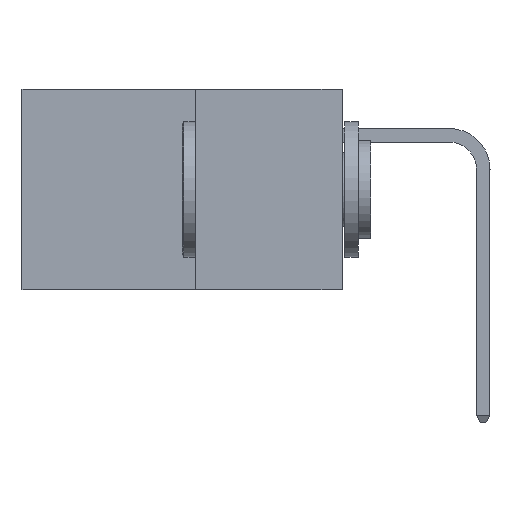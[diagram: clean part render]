
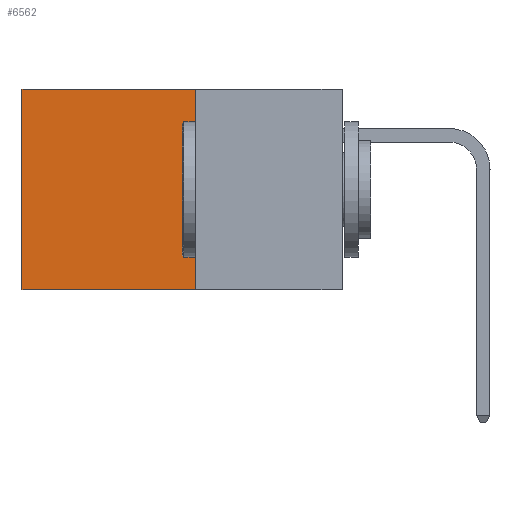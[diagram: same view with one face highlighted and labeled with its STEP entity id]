
A CAD part, left-side view. The second image highlights one B-rep face of the part: STEP entity #6562.
In plain terms, the highlighted planar face has unit normal (-1, 0, 0).
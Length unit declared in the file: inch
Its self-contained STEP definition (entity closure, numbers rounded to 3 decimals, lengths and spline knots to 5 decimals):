
#25 = CARTESIAN_POINT ( 'NONE',  ( 0.277, 0.27, -0.37 ) ) ;
#29 = LINE ( 'NONE', #4669, #7481 ) ;
#82 = DIRECTION ( 'NONE',  ( 0., 0., -1. ) ) ;
#165 = LINE ( 'NONE', #6528, #9218 ) ;
#208 = CARTESIAN_POINT ( 'NONE',  ( 0.277, 0.27, 0. ) ) ;
#1221 = VERTEX_POINT ( 'NONE', #7342 ) ;
#1518 = ORIENTED_EDGE ( 'NONE', *, *, #8991, .F. ) ;
#1585 = CARTESIAN_POINT ( 'NONE',  ( 0.277, 0.27, -0.37 ) ) ;
#2107 = CARTESIAN_POINT ( 'NONE',  ( 0.277, 0.59, -0.37 ) ) ;
#2248 = CARTESIAN_POINT ( 'NONE',  ( 0.277, 0.59, 0. ) ) ;
#2846 = CARTESIAN_POINT ( 'NONE',  ( 0.277, 0.59, -0.37 ) ) ;
#2907 = EDGE_CURVE ( 'NONE', #7593, #7611, #29, .T. ) ;
#4214 = EDGE_CURVE ( 'NONE', #1221, #11573, #5354, .T. ) ;
#4432 = DIRECTION ( 'NONE',  ( 1., 0., 0. ) ) ;
#4669 = CARTESIAN_POINT ( 'NONE',  ( 0.277, 0.27, 0. ) ) ;
#5060 = DIRECTION ( 'NONE',  ( 0., 1., 0. ) ) ;
#5354 = LINE ( 'NONE', #25, #7894 ) ;
#5615 = DIRECTION ( 'NONE',  ( 0., 0., -1. ) ) ;
#5915 = VECTOR ( 'NONE', #82, 39.37008 ) ;
#6528 = CARTESIAN_POINT ( 'NONE',  ( 0.277, 0.27, -0.37 ) ) ;
#6562 = ADVANCED_FACE ( 'NONE', ( #10957 ), #10112, .F. ) ;
#7342 = CARTESIAN_POINT ( 'NONE',  ( 0.277, 0.27, -0.37 ) ) ;
#7481 = VECTOR ( 'NONE', #5060, 39.37008 ) ;
#7593 = VERTEX_POINT ( 'NONE', #208 ) ;
#7611 = VERTEX_POINT ( 'NONE', #2248 ) ;
#7814 = ORIENTED_EDGE ( 'NONE', *, *, #2907, .T. ) ;
#7894 = VECTOR ( 'NONE', #9561, 39.37008 ) ;
#8294 = ORIENTED_EDGE ( 'NONE', *, *, #9733, .T. ) ;
#8991 = EDGE_CURVE ( 'NONE', #7593, #1221, #165, .T. ) ;
#9030 = EDGE_LOOP ( 'NONE', ( #8294, #11590, #1518, #7814 ) ) ;
#9218 = VECTOR ( 'NONE', #5615, 39.37008 ) ;
#9561 = DIRECTION ( 'NONE',  ( 0., 1., 0. ) ) ;
#9733 = EDGE_CURVE ( 'NONE', #7611, #11573, #10869, .T. ) ;
#10112 = PLANE ( 'NONE',  #12219 ) ;
#10869 = LINE ( 'NONE', #2107, #5915 ) ;
#10957 = FACE_OUTER_BOUND ( 'NONE', #9030, .T. ) ;
#11003 = DIRECTION ( 'NONE',  ( 0., 0., -1. ) ) ;
#11573 = VERTEX_POINT ( 'NONE', #2846 ) ;
#11590 = ORIENTED_EDGE ( 'NONE', *, *, #4214, .F. ) ;
#12219 = AXIS2_PLACEMENT_3D ( 'NONE', #1585, #4432, #11003 ) ;
